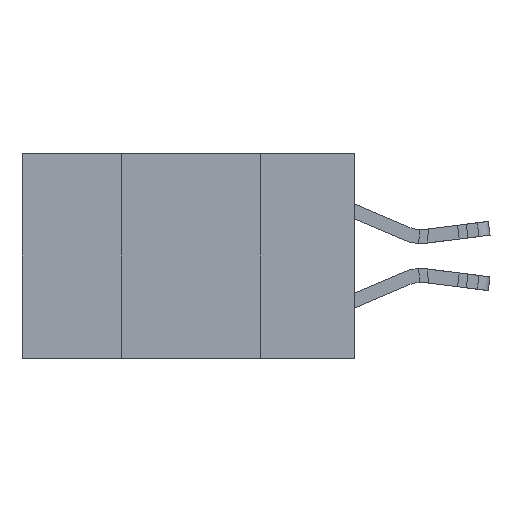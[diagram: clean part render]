
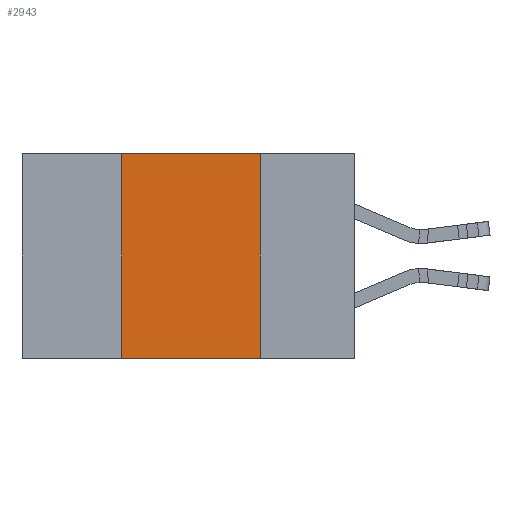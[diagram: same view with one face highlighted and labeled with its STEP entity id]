
A CAD part, left-side view. The second image highlights one B-rep face of the part: STEP entity #2943.
In plain terms, the highlighted planar face has unit normal (-1, 0, 0).
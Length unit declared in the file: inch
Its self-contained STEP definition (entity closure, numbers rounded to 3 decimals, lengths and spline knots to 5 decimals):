
#852 = ORIENTED_EDGE ( 'NONE', *, *, #3796, .F. ) ;
#1995 = DIRECTION ( 'NONE',  ( 0., -1., 0. ) ) ;
#2135 = LINE ( 'NONE', #28369, #13310 ) ;
#2468 = AXIS2_PLACEMENT_3D ( 'NONE', #28338, #12161, #10583 ) ;
#2943 = ADVANCED_FACE ( 'NONE', ( #16922 ), #5118, .F. ) ;
#3484 = VECTOR ( 'NONE', #9378, 39.37008 ) ;
#3796 = EDGE_CURVE ( 'NONE', #14039, #25831, #4613, .T. ) ;
#4299 = DIRECTION ( 'NONE',  ( 0., -1., 0. ) ) ;
#4392 = CARTESIAN_POINT ( 'NONE',  ( 0., 0.6, -0.37 ) ) ;
#4613 = LINE ( 'NONE', #9596, #16435 ) ;
#4663 = VERTEX_POINT ( 'NONE', #15545 ) ;
#5118 = PLANE ( 'NONE',  #2468 ) ;
#6949 = CARTESIAN_POINT ( 'NONE',  ( 0., 0.17, -0.37 ) ) ;
#7063 = DIRECTION ( 'NONE',  ( 0., 0., 1. ) ) ;
#8171 = EDGE_CURVE ( 'NONE', #14039, #26120, #28406, .T. ) ;
#9378 = DIRECTION ( 'NONE',  ( 0., 0., -1. ) ) ;
#9596 = CARTESIAN_POINT ( 'NONE',  ( 0., 0.42, 0. ) ) ;
#10504 = ORIENTED_EDGE ( 'NONE', *, *, #8171, .T. ) ;
#10583 = DIRECTION ( 'NONE',  ( 0., 0., -1. ) ) ;
#12161 = DIRECTION ( 'NONE',  ( 1., 0., 0. ) ) ;
#13284 = EDGE_CURVE ( 'NONE', #25831, #4663, #2135, .T. ) ;
#13310 = VECTOR ( 'NONE', #1995, 39.37008 ) ;
#14039 = VERTEX_POINT ( 'NONE', #26290 ) ;
#14651 = ORIENTED_EDGE ( 'NONE', *, *, #13284, .F. ) ;
#15545 = CARTESIAN_POINT ( 'NONE',  ( 0., 0.17, 0. ) ) ;
#16435 = VECTOR ( 'NONE', #7063, 39.37008 ) ;
#16922 = FACE_OUTER_BOUND ( 'NONE', #25594, .T. ) ;
#20507 = LINE ( 'NONE', #24769, #3484 ) ;
#21761 = ORIENTED_EDGE ( 'NONE', *, *, #24156, .F. ) ;
#22685 = VECTOR ( 'NONE', #4299, 39.37008 ) ;
#24156 = EDGE_CURVE ( 'NONE', #4663, #26120, #20507, .T. ) ;
#24769 = CARTESIAN_POINT ( 'NONE',  ( 0., 0.17, 0. ) ) ;
#25594 = EDGE_LOOP ( 'NONE', ( #21761, #14651, #852, #10504 ) ) ;
#25831 = VERTEX_POINT ( 'NONE', #27867 ) ;
#26120 = VERTEX_POINT ( 'NONE', #6949 ) ;
#26290 = CARTESIAN_POINT ( 'NONE',  ( 0., 0.42, -0.37 ) ) ;
#27867 = CARTESIAN_POINT ( 'NONE',  ( 0., 0.42, 0. ) ) ;
#28338 = CARTESIAN_POINT ( 'NONE',  ( 0., 0.6, 0. ) ) ;
#28369 = CARTESIAN_POINT ( 'NONE',  ( 0., 0.6, 0. ) ) ;
#28406 = LINE ( 'NONE', #4392, #22685 ) ;
